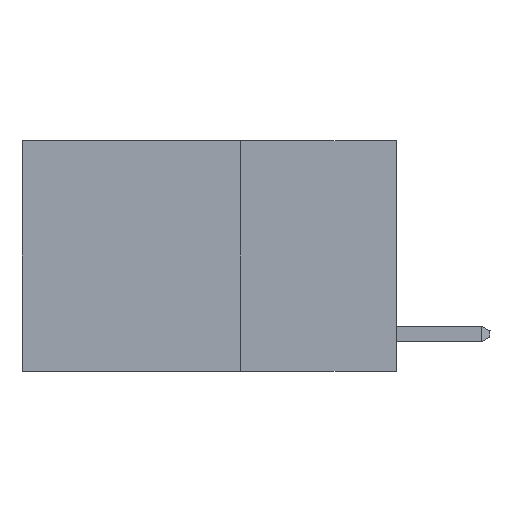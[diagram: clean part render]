
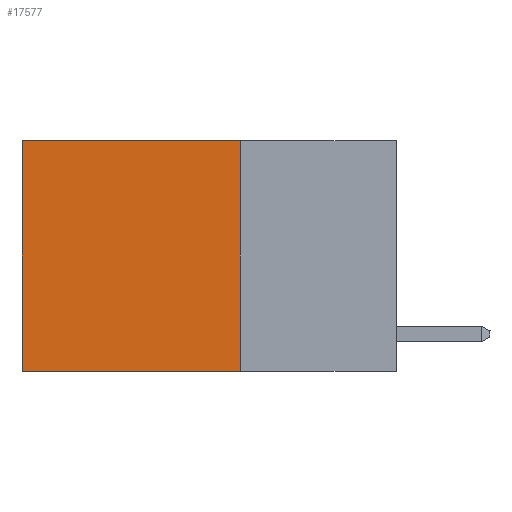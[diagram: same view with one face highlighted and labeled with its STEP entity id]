
A CAD part, left-side view. The second image highlights one B-rep face of the part: STEP entity #17577.
In plain terms, the highlighted planar face has unit normal (-1, 0, 0).
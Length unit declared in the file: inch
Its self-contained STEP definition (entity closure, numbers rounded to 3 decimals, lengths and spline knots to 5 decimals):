
#213 = VERTEX_POINT ( 'NONE', #17977 ) ;
#505 = EDGE_CURVE ( 'NONE', #6795, #9751, #16305, .T. ) ;
#587 = CARTESIAN_POINT ( 'NONE',  ( 0.2625, 0.6, 0. ) ) ;
#786 = DIRECTION ( 'NONE',  ( 0., 1., 0. ) ) ;
#804 = LINE ( 'NONE', #13285, #12233 ) ;
#885 = EDGE_LOOP ( 'NONE', ( #16974, #9294, #1419, #8584 ) ) ;
#1419 = ORIENTED_EDGE ( 'NONE', *, *, #4407, .F. ) ;
#2081 = VERTEX_POINT ( 'NONE', #5833 ) ;
#2518 = VECTOR ( 'NONE', #786, 39.37008 ) ;
#3186 = AXIS2_PLACEMENT_3D ( 'NONE', #4025, #8012, #13654 ) ;
#3305 = VECTOR ( 'NONE', #5098, 39.37008 ) ;
#3593 = EDGE_CURVE ( 'NONE', #213, #2081, #13872, .T. ) ;
#4025 = CARTESIAN_POINT ( 'NONE',  ( 0.2625, 0.25, 0. ) ) ;
#4407 = EDGE_CURVE ( 'NONE', #213, #6795, #804, .T. ) ;
#4791 = CARTESIAN_POINT ( 'NONE',  ( 0.2625, 0.25, -0.37 ) ) ;
#5098 = DIRECTION ( 'NONE',  ( 0., 1., 0. ) ) ;
#5122 = DIRECTION ( 'NONE',  ( 0., 0., -1. ) ) ;
#5833 = CARTESIAN_POINT ( 'NONE',  ( 0.2625, 0.6, 0. ) ) ;
#6795 = VERTEX_POINT ( 'NONE', #4791 ) ;
#8012 = DIRECTION ( 'NONE',  ( 1., 0., 0. ) ) ;
#8584 = ORIENTED_EDGE ( 'NONE', *, *, #3593, .T. ) ;
#9294 = ORIENTED_EDGE ( 'NONE', *, *, #505, .F. ) ;
#9455 = CARTESIAN_POINT ( 'NONE',  ( 0.2625, 0.25, 0. ) ) ;
#9751 = VERTEX_POINT ( 'NONE', #14501 ) ;
#11057 = PLANE ( 'NONE',  #3186 ) ;
#11881 = CARTESIAN_POINT ( 'NONE',  ( 0.2625, 0.25, -0.37 ) ) ;
#12233 = VECTOR ( 'NONE', #5122, 39.37008 ) ;
#13285 = CARTESIAN_POINT ( 'NONE',  ( 0.2625, 0.25, 0. ) ) ;
#13654 = DIRECTION ( 'NONE',  ( 0., 0., -1. ) ) ;
#13729 = VECTOR ( 'NONE', #17493, 39.37008 ) ;
#13872 = LINE ( 'NONE', #9455, #3305 ) ;
#14501 = CARTESIAN_POINT ( 'NONE',  ( 0.2625, 0.6, -0.37 ) ) ;
#14632 = LINE ( 'NONE', #587, #13729 ) ;
#14726 = EDGE_CURVE ( 'NONE', #2081, #9751, #14632, .T. ) ;
#16305 = LINE ( 'NONE', #11881, #2518 ) ;
#16605 = FACE_OUTER_BOUND ( 'NONE', #885, .T. ) ;
#16974 = ORIENTED_EDGE ( 'NONE', *, *, #14726, .T. ) ;
#17493 = DIRECTION ( 'NONE',  ( 0., 0., -1. ) ) ;
#17577 = ADVANCED_FACE ( 'NONE', ( #16605 ), #11057, .F. ) ;
#17977 = CARTESIAN_POINT ( 'NONE',  ( 0.2625, 0.25, 0. ) ) ;
